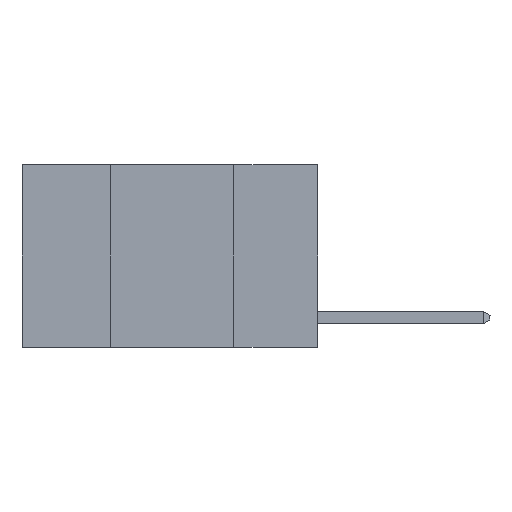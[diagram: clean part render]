
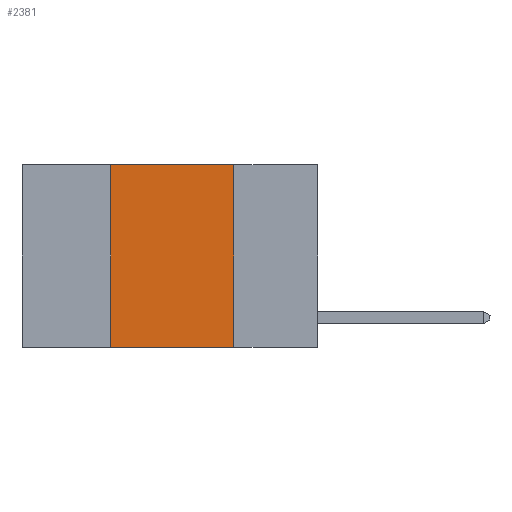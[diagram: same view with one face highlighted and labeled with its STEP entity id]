
A CAD part, left-side view. The second image highlights one B-rep face of the part: STEP entity #2381.
In plain terms, the highlighted planar face has unit normal (-1, 0, 0).
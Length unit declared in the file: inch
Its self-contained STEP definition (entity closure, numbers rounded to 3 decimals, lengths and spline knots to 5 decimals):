
#271 = DIRECTION ( 'NONE',  ( 0., -1., 0. ) ) ;
#623 = CARTESIAN_POINT ( 'NONE',  ( 0., 0.42, -0.37 ) ) ;
#789 = AXIS2_PLACEMENT_3D ( 'NONE', #7997, #5865, #8901 ) ;
#1071 = CARTESIAN_POINT ( 'NONE',  ( 0., 0.6, 0. ) ) ;
#1095 = EDGE_CURVE ( 'NONE', #6597, #1816, #1994, .T. ) ;
#1297 = ORIENTED_EDGE ( 'NONE', *, *, #6542, .T. ) ;
#1816 = VERTEX_POINT ( 'NONE', #9553 ) ;
#1994 = LINE ( 'NONE', #5063, #8344 ) ;
#2381 = ADVANCED_FACE ( 'NONE', ( #3606 ), #2823, .F. ) ;
#2390 = ORIENTED_EDGE ( 'NONE', *, *, #1095, .F. ) ;
#2562 = DIRECTION ( 'NONE',  ( 0., 0., 1. ) ) ;
#2774 = VECTOR ( 'NONE', #3389, 39.37008 ) ;
#2823 = PLANE ( 'NONE',  #789 ) ;
#3246 = EDGE_CURVE ( 'NONE', #6753, #5267, #7787, .T. ) ;
#3389 = DIRECTION ( 'NONE',  ( 0., -1., 0. ) ) ;
#3606 = FACE_OUTER_BOUND ( 'NONE', #7313, .T. ) ;
#3694 = ORIENTED_EDGE ( 'NONE', *, *, #5214, .F. ) ;
#4056 = VECTOR ( 'NONE', #271, 39.37008 ) ;
#4286 = CARTESIAN_POINT ( 'NONE',  ( 0., 0.17, 0. ) ) ;
#4680 = CARTESIAN_POINT ( 'NONE',  ( 0., 0.6, -0.37 ) ) ;
#4882 = VECTOR ( 'NONE', #2562, 39.37008 ) ;
#5058 = ORIENTED_EDGE ( 'NONE', *, *, #3246, .F. ) ;
#5063 = CARTESIAN_POINT ( 'NONE',  ( 0., 0.17, 0. ) ) ;
#5214 = EDGE_CURVE ( 'NONE', #5267, #6597, #7933, .T. ) ;
#5267 = VERTEX_POINT ( 'NONE', #8233 ) ;
#5865 = DIRECTION ( 'NONE',  ( 1., 0., 0. ) ) ;
#6542 = EDGE_CURVE ( 'NONE', #6753, #1816, #9328, .T. ) ;
#6597 = VERTEX_POINT ( 'NONE', #4286 ) ;
#6753 = VERTEX_POINT ( 'NONE', #623 ) ;
#7313 = EDGE_LOOP ( 'NONE', ( #2390, #3694, #5058, #1297 ) ) ;
#7787 = LINE ( 'NONE', #9223, #4882 ) ;
#7933 = LINE ( 'NONE', #1071, #2774 ) ;
#7997 = CARTESIAN_POINT ( 'NONE',  ( 0., 0.6, 0. ) ) ;
#8100 = DIRECTION ( 'NONE',  ( 0., 0., -1. ) ) ;
#8233 = CARTESIAN_POINT ( 'NONE',  ( 0., 0.42, 0. ) ) ;
#8344 = VECTOR ( 'NONE', #8100, 39.37008 ) ;
#8901 = DIRECTION ( 'NONE',  ( 0., 0., -1. ) ) ;
#9223 = CARTESIAN_POINT ( 'NONE',  ( 0., 0.42, 0. ) ) ;
#9328 = LINE ( 'NONE', #4680, #4056 ) ;
#9553 = CARTESIAN_POINT ( 'NONE',  ( 0., 0.17, -0.37 ) ) ;
